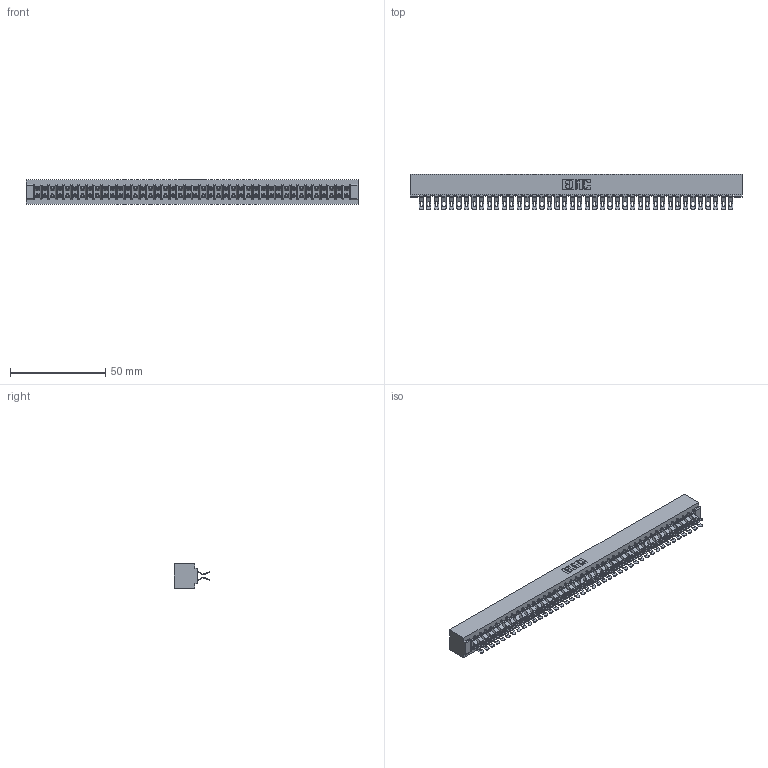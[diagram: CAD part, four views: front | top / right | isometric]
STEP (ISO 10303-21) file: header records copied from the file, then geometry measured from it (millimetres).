
FILE_DESCRIPTION (( 'STEP AP203' ), '1' );
FILE_NAME ('357-084-555-201.STEP', '2019-09-19T18:04:57', ( '' ), ( '' ), 'SwSTEP 2.0', 'SolidWorks 2016', '' );
FILE_SCHEMA (( 'CONFIG_CONTROL_DESIGN' ));
Length unit declared in the file: inch
Products named in the file (3): 357-084-555-201; 307 Part_No Mounting Lugs; 307-290-001_555
Assembly tree (85 placements, depth 2):
  357-084-555-201
    307 Part_No Mounting Lugs
    307-290-001_555  x84
Bounding box: 174.29 x 18.75 x 12.7 mm (x, y, z)
Volume: 19332 mm3; surface area: 25357.8 mm2
Topology: 85 solids, 85 shells, 5277 faces, 15503 edges, 10106 vertices
Faces by surface type: plane 2922, cylinder 2269, sphere 86
Entity records: 37609 total; most frequent: CARTESIAN_POINT 6154, ORIENTED_EDGE 6100, DIRECTION 6034, EDGE_CURVE 3050, VECTOR 2330, LINE 2330, VERTEX_POINT 1972, AXIS2_PLACEMENT_3D 1852
